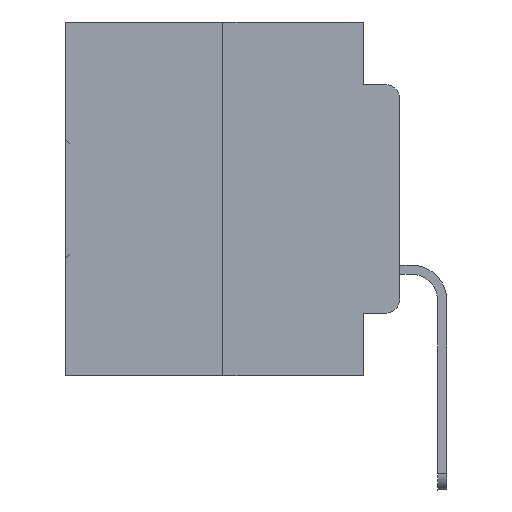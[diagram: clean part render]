
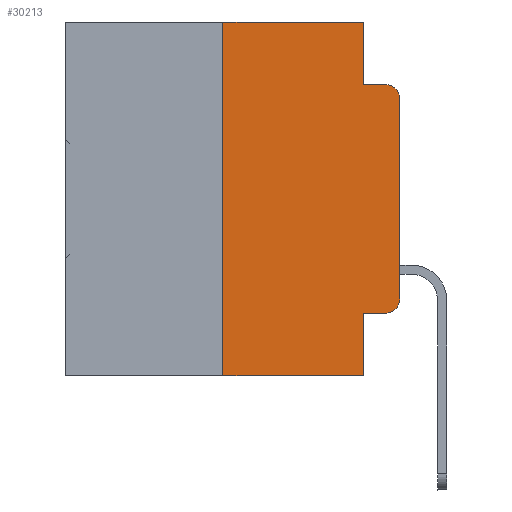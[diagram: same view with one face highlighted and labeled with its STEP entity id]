
A CAD part, left-side view. The second image highlights one B-rep face of the part: STEP entity #30213.
In plain terms, the highlighted planar face has unit normal (-1, 0, 0).
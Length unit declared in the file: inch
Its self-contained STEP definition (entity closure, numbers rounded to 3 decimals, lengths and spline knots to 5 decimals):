
#190 = VERTEX_POINT ( 'NONE', #27831 ) ;
#344 = EDGE_LOOP ( 'NONE', ( #29930, #17065, #22219, #22671, #16060, #6196, #12715, #20906, #16435, #1849 ) ) ;
#413 = DIRECTION ( 'NONE',  ( 0., -1., 0. ) ) ;
#447 = EDGE_CURVE ( 'NONE', #190, #4627, #18666, .T. ) ;
#682 = DIRECTION ( 'NONE',  ( 0., 0., -1. ) ) ;
#1660 = DIRECTION ( 'NONE',  ( 0., -1., 0. ) ) ;
#1849 = ORIENTED_EDGE ( 'NONE', *, *, #18185, .T. ) ;
#1868 = PLANE ( 'NONE',  #12763 ) ;
#2614 = CARTESIAN_POINT ( 'NONE',  ( 0., 0.051, 0. ) ) ;
#2664 = EDGE_CURVE ( 'NONE', #13924, #17715, #24533, .T. ) ;
#2762 = CARTESIAN_POINT ( 'NONE',  ( 0., 0.25, 0. ) ) ;
#3421 = DIRECTION ( 'NONE',  ( -1., 0., 0. ) ) ;
#3618 = VECTOR ( 'NONE', #1660, 39.37008 ) ;
#3827 = DIRECTION ( 'NONE',  ( 0., -1., 0. ) ) ;
#4232 = CARTESIAN_POINT ( 'NONE',  ( 0., 0.051, -0.0885 ) ) ;
#4272 = DIRECTION ( 'NONE',  ( 1., 0., 0. ) ) ;
#4627 = VERTEX_POINT ( 'NONE', #11300 ) ;
#4819 = CARTESIAN_POINT ( 'NONE',  ( 0., 0.473, 0. ) ) ;
#5194 = DIRECTION ( 'NONE',  ( 0., 0., 1. ) ) ;
#6196 = ORIENTED_EDGE ( 'NONE', *, *, #21051, .F. ) ;
#6556 = CIRCLE ( 'NONE', #24466, 0.02 ) ;
#6703 = DIRECTION ( 'NONE',  ( 0., 0., -1. ) ) ;
#7434 = LINE ( 'NONE', #2762, #8000 ) ;
#7610 = VECTOR ( 'NONE', #9811, 39.37008 ) ;
#7641 = CARTESIAN_POINT ( 'NONE',  ( 0., 0.051, 0. ) ) ;
#8000 = VECTOR ( 'NONE', #5194, 39.37008 ) ;
#8631 = EDGE_CURVE ( 'NONE', #30181, #4627, #15065, .T. ) ;
#9165 = CARTESIAN_POINT ( 'NONE',  ( 0., 0.051, -0.4115 ) ) ;
#9811 = DIRECTION ( 'NONE',  ( 0., -1., 0. ) ) ;
#10057 = DIRECTION ( 'NONE',  ( 0., 0., -1. ) ) ;
#10254 = LINE ( 'NONE', #24831, #30531 ) ;
#10493 = CARTESIAN_POINT ( 'NONE',  ( 0., 0.02, -0.3915 ) ) ;
#11300 = CARTESIAN_POINT ( 'NONE',  ( 0., 0.02, -0.0885 ) ) ;
#12338 = DIRECTION ( 'NONE',  ( 0., 0., -1. ) ) ;
#12715 = ORIENTED_EDGE ( 'NONE', *, *, #12745, .T. ) ;
#12745 = EDGE_CURVE ( 'NONE', #26351, #17715, #22551, .T. ) ;
#12763 = AXIS2_PLACEMENT_3D ( 'NONE', #31063, #4272, #6703 ) ;
#12769 = CARTESIAN_POINT ( 'NONE',  ( 0., 0.02, -0.4115 ) ) ;
#12772 = CARTESIAN_POINT ( 'NONE',  ( 0., 0.02, -0.1085 ) ) ;
#13141 = VERTEX_POINT ( 'NONE', #20268 ) ;
#13924 = VERTEX_POINT ( 'NONE', #9165 ) ;
#14817 = VECTOR ( 'NONE', #12338, 39.37008 ) ;
#15065 = CIRCLE ( 'NONE', #19684, 0.02 ) ;
#15343 = DIRECTION ( 'NONE',  ( -1., 0., 0. ) ) ;
#15688 = CARTESIAN_POINT ( 'NONE',  ( 0., 0., -0.1085 ) ) ;
#16060 = ORIENTED_EDGE ( 'NONE', *, *, #23996, .F. ) ;
#16435 = ORIENTED_EDGE ( 'NONE', *, *, #19878, .T. ) ;
#17065 = ORIENTED_EDGE ( 'NONE', *, *, #8631, .T. ) ;
#17304 = DIRECTION ( 'NONE',  ( 0., 0., 1. ) ) ;
#17434 = CARTESIAN_POINT ( 'NONE',  ( 0., 0.473, -0.5 ) ) ;
#17555 = LINE ( 'NONE', #7641, #24937 ) ;
#17657 = CARTESIAN_POINT ( 'NONE',  ( 0., 0., -0.3915 ) ) ;
#17715 = VERTEX_POINT ( 'NONE', #22581 ) ;
#17733 = CARTESIAN_POINT ( 'NONE',  ( 0., 0.25, -0.5 ) ) ;
#18185 = EDGE_CURVE ( 'NONE', #26304, #18621, #6556, .T. ) ;
#18621 = VERTEX_POINT ( 'NONE', #17657 ) ;
#18666 = LINE ( 'NONE', #4232, #3618 ) ;
#19122 = VECTOR ( 'NONE', #3827, 39.37008 ) ;
#19684 = AXIS2_PLACEMENT_3D ( 'NONE', #12772, #15343, #10057 ) ;
#19878 = EDGE_CURVE ( 'NONE', #13924, #26304, #29825, .T. ) ;
#20268 = CARTESIAN_POINT ( 'NONE',  ( 0., 0.25, 0. ) ) ;
#20687 = EDGE_CURVE ( 'NONE', #30902, #190, #17555, .T. ) ;
#20906 = ORIENTED_EDGE ( 'NONE', *, *, #2664, .F. ) ;
#21051 = EDGE_CURVE ( 'NONE', #26351, #13141, #7434, .T. ) ;
#21289 = VECTOR ( 'NONE', #413, 39.37008 ) ;
#22098 = CARTESIAN_POINT ( 'NONE',  ( 0., 0.051, 0. ) ) ;
#22117 = LINE ( 'NONE', #4819, #7610 ) ;
#22219 = ORIENTED_EDGE ( 'NONE', *, *, #447, .F. ) ;
#22551 = LINE ( 'NONE', #17434, #21289 ) ;
#22581 = CARTESIAN_POINT ( 'NONE',  ( 0., 0.051, -0.5 ) ) ;
#22671 = ORIENTED_EDGE ( 'NONE', *, *, #20687, .F. ) ;
#23996 = EDGE_CURVE ( 'NONE', #13141, #30902, #22117, .T. ) ;
#24466 = AXIS2_PLACEMENT_3D ( 'NONE', #10493, #3421, #682 ) ;
#24533 = LINE ( 'NONE', #22098, #14817 ) ;
#24831 = CARTESIAN_POINT ( 'NONE',  ( 0., 0., 0. ) ) ;
#24937 = VECTOR ( 'NONE', #27339, 39.37008 ) ;
#25029 = CARTESIAN_POINT ( 'NONE',  ( 0., 0.051, -0.4115 ) ) ;
#26304 = VERTEX_POINT ( 'NONE', #12769 ) ;
#26351 = VERTEX_POINT ( 'NONE', #17733 ) ;
#26400 = FACE_OUTER_BOUND ( 'NONE', #344, .T. ) ;
#27042 = EDGE_CURVE ( 'NONE', #18621, #30181, #10254, .T. ) ;
#27339 = DIRECTION ( 'NONE',  ( 0., 0., -1. ) ) ;
#27831 = CARTESIAN_POINT ( 'NONE',  ( 0., 0.051, -0.0885 ) ) ;
#29825 = LINE ( 'NONE', #25029, #19122 ) ;
#29930 = ORIENTED_EDGE ( 'NONE', *, *, #27042, .T. ) ;
#30181 = VERTEX_POINT ( 'NONE', #15688 ) ;
#30213 = ADVANCED_FACE ( 'NONE', ( #26400 ), #1868, .F. ) ;
#30531 = VECTOR ( 'NONE', #17304, 39.37008 ) ;
#30902 = VERTEX_POINT ( 'NONE', #2614 ) ;
#31063 = CARTESIAN_POINT ( 'NONE',  ( 0., 0.473, 0. ) ) ;
